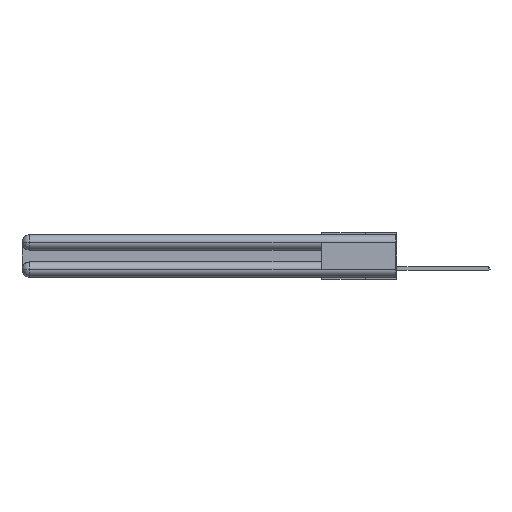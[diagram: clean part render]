
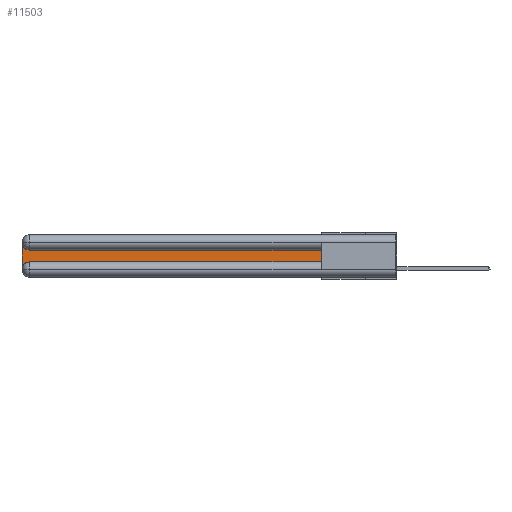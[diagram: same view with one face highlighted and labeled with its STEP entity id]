
A CAD part, left-side view. The second image highlights one B-rep face of the part: STEP entity #11503.
In plain terms, the highlighted planar face has unit normal (-1, 0, 0).
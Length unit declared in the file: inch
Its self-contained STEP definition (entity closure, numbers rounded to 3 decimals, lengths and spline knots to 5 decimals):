
#353 = DIRECTION ( 'NONE',  ( 1., 0., 0. ) ) ;
#1978 = AXIS2_PLACEMENT_3D ( 'NONE', #4508, #22717, #18263 ) ;
#2617 = ORIENTED_EDGE ( 'NONE', *, *, #13221, .T. ) ;
#2885 = CARTESIAN_POINT ( 'NONE',  ( 0.075, 3., -0.2175 ) ) ;
#3310 = CARTESIAN_POINT ( 'NONE',  ( 0.075, 0.6, -0.1225 ) ) ;
#3911 = DIRECTION ( 'NONE',  ( 0., 0., -1. ) ) ;
#4300 = AXIS2_PLACEMENT_3D ( 'NONE', #7596, #353, #23672 ) ;
#4508 = CARTESIAN_POINT ( 'NONE',  ( 0.075, 2.94, -0.2775 ) ) ;
#4741 = DIRECTION ( 'NONE',  ( 0., -1., 0. ) ) ;
#6322 = VERTEX_POINT ( 'NONE', #8777 ) ;
#6984 = DIRECTION ( 'NONE',  ( 0., 0., 1. ) ) ;
#7596 = CARTESIAN_POINT ( 'NONE',  ( 0.075, 2.94, -0.0625 ) ) ;
#8587 = VERTEX_POINT ( 'NONE', #13830 ) ;
#8623 = VERTEX_POINT ( 'NONE', #11614 ) ;
#8777 = CARTESIAN_POINT ( 'NONE',  ( 0.075, 2.94, -0.2175 ) ) ;
#8871 = CARTESIAN_POINT ( 'NONE',  ( 0.075, 0.6, -0.1225 ) ) ;
#9351 = CARTESIAN_POINT ( 'NONE',  ( 0.075, 3., -0.1225 ) ) ;
#9621 = EDGE_CURVE ( 'NONE', #8623, #13831, #24279, .T. ) ;
#9771 = ORIENTED_EDGE ( 'NONE', *, *, #14171, .T. ) ;
#11503 = ADVANCED_FACE ( 'NONE', ( #18000 ), #20738, .F. ) ;
#11614 = CARTESIAN_POINT ( 'NONE',  ( 0.075, 0.6, -0.2175 ) ) ;
#12557 = ORIENTED_EDGE ( 'NONE', *, *, #14122, .T. ) ;
#12996 = CARTESIAN_POINT ( 'NONE',  ( 0.075, 3., -0.0625 ) ) ;
#13221 = EDGE_CURVE ( 'NONE', #8587, #20389, #14676, .T. ) ;
#13830 = CARTESIAN_POINT ( 'NONE',  ( 0.075, 2.94, -0.1225 ) ) ;
#13831 = VERTEX_POINT ( 'NONE', #3310 ) ;
#13917 = LINE ( 'NONE', #25473, #16455 ) ;
#14122 = EDGE_CURVE ( 'NONE', #18249, #6322, #27359, .T. ) ;
#14171 = EDGE_CURVE ( 'NONE', #13831, #8587, #20423, .T. ) ;
#14227 = VECTOR ( 'NONE', #27516, 39.37008 ) ;
#14676 = CIRCLE ( 'NONE', #4300, 0.06 ) ;
#15305 = ORIENTED_EDGE ( 'NONE', *, *, #19485, .T. ) ;
#16163 = DIRECTION ( 'NONE',  ( 1., 0., 0. ) ) ;
#16269 = DIRECTION ( 'NONE',  ( 0., 0., -1. ) ) ;
#16455 = VECTOR ( 'NONE', #4741, 39.37008 ) ;
#18000 = FACE_OUTER_BOUND ( 'NONE', #28296, .T. ) ;
#18249 = VERTEX_POINT ( 'NONE', #18657 ) ;
#18263 = DIRECTION ( 'NONE',  ( 0., 0., -1. ) ) ;
#18657 = CARTESIAN_POINT ( 'NONE',  ( 0.075, 3., -0.2775 ) ) ;
#19485 = EDGE_CURVE ( 'NONE', #6322, #8623, #13917, .T. ) ;
#20389 = VERTEX_POINT ( 'NONE', #12996 ) ;
#20423 = LINE ( 'NONE', #8871, #14227 ) ;
#20738 = PLANE ( 'NONE',  #29646 ) ;
#21319 = EDGE_CURVE ( 'NONE', #20389, #18249, #29805, .T. ) ;
#22125 = ORIENTED_EDGE ( 'NONE', *, *, #9621, .T. ) ;
#22717 = DIRECTION ( 'NONE',  ( 1., 0., 0. ) ) ;
#23541 = VECTOR ( 'NONE', #6984, 39.37008 ) ;
#23672 = DIRECTION ( 'NONE',  ( 0., 0., -1. ) ) ;
#24279 = LINE ( 'NONE', #30213, #23541 ) ;
#25473 = CARTESIAN_POINT ( 'NONE',  ( 0.075, 0.6, -0.2175 ) ) ;
#26966 = ORIENTED_EDGE ( 'NONE', *, *, #21319, .T. ) ;
#27359 = CIRCLE ( 'NONE', #1978, 0.06 ) ;
#27516 = DIRECTION ( 'NONE',  ( 0., 1., 0. ) ) ;
#28296 = EDGE_LOOP ( 'NONE', ( #9771, #2617, #26966, #12557, #15305, #22125 ) ) ;
#28714 = VECTOR ( 'NONE', #3911, 39.37008 ) ;
#29646 = AXIS2_PLACEMENT_3D ( 'NONE', #9351, #16163, #16269 ) ;
#29805 = LINE ( 'NONE', #2885, #28714 ) ;
#30213 = CARTESIAN_POINT ( 'NONE',  ( 0.075, 0.6, -0.2175 ) ) ;
